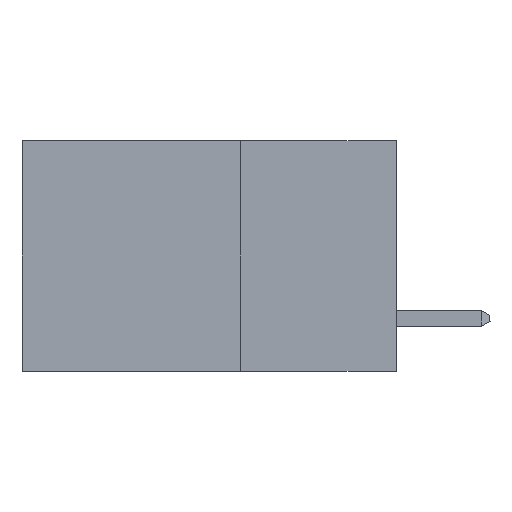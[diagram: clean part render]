
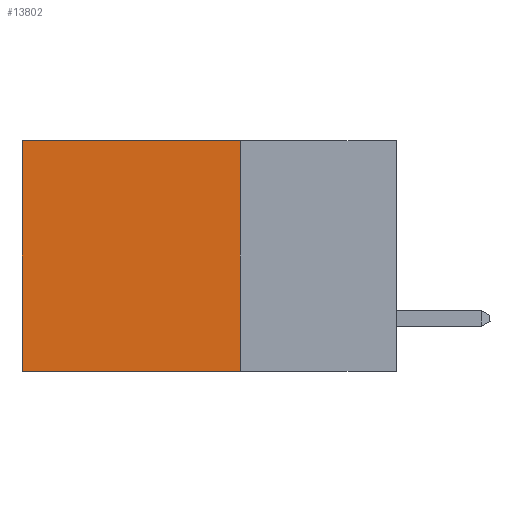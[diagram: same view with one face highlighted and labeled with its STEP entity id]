
A CAD part, left-side view. The second image highlights one B-rep face of the part: STEP entity #13802.
In plain terms, the highlighted planar face has unit normal (-1, 0, 0).
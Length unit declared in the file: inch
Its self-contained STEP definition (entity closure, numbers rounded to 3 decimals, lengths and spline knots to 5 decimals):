
#456 = FACE_OUTER_BOUND ( 'NONE', #7440, .T. ) ;
#1721 = ORIENTED_EDGE ( 'NONE', *, *, #13705, .F. ) ;
#2100 = EDGE_CURVE ( 'NONE', #2553, #19656, #3494, .T. ) ;
#2162 = AXIS2_PLACEMENT_3D ( 'NONE', #14897, #13306, #13490 ) ;
#2460 = CARTESIAN_POINT ( 'NONE',  ( 0.298, 0.6, -0.37 ) ) ;
#2553 = VERTEX_POINT ( 'NONE', #9343 ) ;
#3146 = VECTOR ( 'NONE', #24432, 39.37008 ) ;
#3369 = VERTEX_POINT ( 'NONE', #25886 ) ;
#3451 = VECTOR ( 'NONE', #17741, 39.37008 ) ;
#3494 = LINE ( 'NONE', #9191, #3146 ) ;
#4235 = LINE ( 'NONE', #16994, #15104 ) ;
#5802 = CARTESIAN_POINT ( 'NONE',  ( 0.298, 0.25, -0.37 ) ) ;
#7097 = CARTESIAN_POINT ( 'NONE',  ( 0.298, 0.6, 0. ) ) ;
#7440 = EDGE_LOOP ( 'NONE', ( #16080, #26820, #1721, #8447 ) ) ;
#8239 = CARTESIAN_POINT ( 'NONE',  ( 0.298, 0.6, 0. ) ) ;
#8447 = ORIENTED_EDGE ( 'NONE', *, *, #2100, .T. ) ;
#9186 = PLANE ( 'NONE',  #2162 ) ;
#9191 = CARTESIAN_POINT ( 'NONE',  ( 0.298, 0.25, 0. ) ) ;
#9343 = CARTESIAN_POINT ( 'NONE',  ( 0.298, 0.25, 0. ) ) ;
#10582 = LINE ( 'NONE', #7097, #3451 ) ;
#10940 = EDGE_CURVE ( 'NONE', #3369, #13847, #18856, .T. ) ;
#13306 = DIRECTION ( 'NONE',  ( 1., 0., 0. ) ) ;
#13490 = DIRECTION ( 'NONE',  ( 0., 0., -1. ) ) ;
#13705 = EDGE_CURVE ( 'NONE', #2553, #3369, #4235, .T. ) ;
#13802 = ADVANCED_FACE ( 'NONE', ( #456 ), #9186, .F. ) ;
#13847 = VERTEX_POINT ( 'NONE', #2460 ) ;
#14530 = DIRECTION ( 'NONE',  ( 0., 0., -1. ) ) ;
#14897 = CARTESIAN_POINT ( 'NONE',  ( 0.298, 0.25, 0. ) ) ;
#15104 = VECTOR ( 'NONE', #14530, 39.37008 ) ;
#15785 = VECTOR ( 'NONE', #16629, 39.37008 ) ;
#16080 = ORIENTED_EDGE ( 'NONE', *, *, #20755, .T. ) ;
#16629 = DIRECTION ( 'NONE',  ( 0., 1., 0. ) ) ;
#16994 = CARTESIAN_POINT ( 'NONE',  ( 0.298, 0.25, 0. ) ) ;
#17741 = DIRECTION ( 'NONE',  ( 0., 0., -1. ) ) ;
#18856 = LINE ( 'NONE', #5802, #15785 ) ;
#19656 = VERTEX_POINT ( 'NONE', #8239 ) ;
#20755 = EDGE_CURVE ( 'NONE', #19656, #13847, #10582, .T. ) ;
#24432 = DIRECTION ( 'NONE',  ( 0., 1., 0. ) ) ;
#25886 = CARTESIAN_POINT ( 'NONE',  ( 0.298, 0.25, -0.37 ) ) ;
#26820 = ORIENTED_EDGE ( 'NONE', *, *, #10940, .F. ) ;
